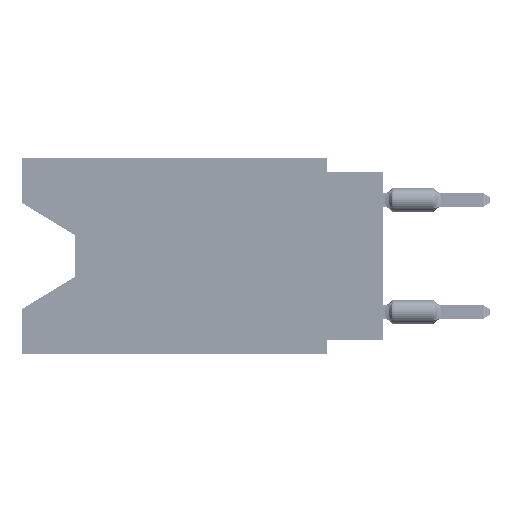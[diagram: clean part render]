
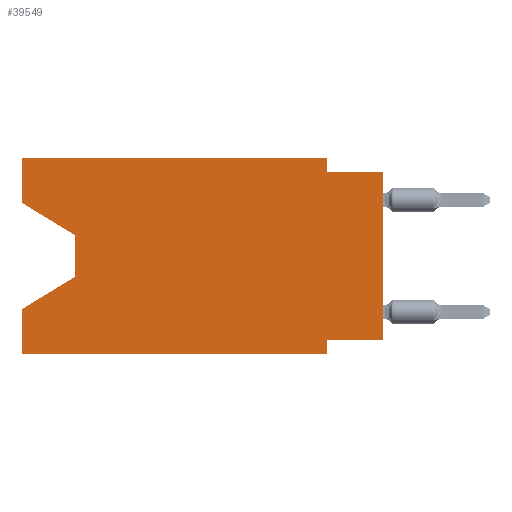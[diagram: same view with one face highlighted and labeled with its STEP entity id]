
A CAD part, left-side view. The second image highlights one B-rep face of the part: STEP entity #39549.
In plain terms, the highlighted planar face has unit normal (-1, 0, 0).
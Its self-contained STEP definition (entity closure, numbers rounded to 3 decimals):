
#186 = CARTESIAN_POINT ( 'NONE',  ( 0., 13.97, -3.505 ) ) ;
#705 = VECTOR ( 'NONE', #32725, 1000. ) ;
#3178 = LINE ( 'NONE', #24293, #705 ) ;
#3574 = EDGE_CURVE ( 'NONE', #90487, #19318, #28671, .T. ) ;
#4982 = LINE ( 'NONE', #40640, #40463 ) ;
#5003 = ORIENTED_EDGE ( 'NONE', *, *, #71803, .F. ) ;
#5248 = VECTOR ( 'NONE', #91007, 1000. ) ;
#5415 = AXIS2_PLACEMENT_3D ( 'NONE', #37842, #21470, #50098 ) ;
#6833 = EDGE_CURVE ( 'NONE', #45487, #69185, #16198, .T. ) ;
#7172 = CARTESIAN_POINT ( 'NONE',  ( 0., 0., 0. ) ) ;
#7627 = DIRECTION ( 'NONE',  ( 0., 0., 1. ) ) ;
#7762 = DIRECTION ( 'NONE',  ( 0., -1., 0. ) ) ;
#8954 = VERTEX_POINT ( 'NONE', #88447 ) ;
#8964 = DIRECTION ( 'NONE',  ( 0., -1., 0. ) ) ;
#9217 = FACE_OUTER_BOUND ( 'NONE', #57411, .T. ) ;
#9561 = CARTESIAN_POINT ( 'NONE',  ( 0., 2.54, 0. ) ) ;
#10021 = CARTESIAN_POINT ( 'NONE',  ( 0., 2.54, -0.635 ) ) ;
#10395 = ORIENTED_EDGE ( 'NONE', *, *, #75110, .F. ) ;
#11474 = CARTESIAN_POINT ( 'NONE',  ( 0., 16.383, -8.89 ) ) ;
#11781 = CARTESIAN_POINT ( 'NONE',  ( 0., 16.383, -2.038 ) ) ;
#15546 = ORIENTED_EDGE ( 'NONE', *, *, #28609, .F. ) ;
#16198 = LINE ( 'NONE', #44834, #74583 ) ;
#16408 = VERTEX_POINT ( 'NONE', #62722 ) ;
#18601 = DIRECTION ( 'NONE',  ( 0., 0., -1. ) ) ;
#19318 = VERTEX_POINT ( 'NONE', #81141 ) ;
#19736 = CARTESIAN_POINT ( 'NONE',  ( 0., 16.383, -2.038 ) ) ;
#19882 = VERTEX_POINT ( 'NONE', #11474 ) ;
#19890 = ORIENTED_EDGE ( 'NONE', *, *, #6833, .F. ) ;
#20108 = VECTOR ( 'NONE', #28737, 1000. ) ;
#21470 = DIRECTION ( 'NONE',  ( 1., 0., 0. ) ) ;
#22603 = ORIENTED_EDGE ( 'NONE', *, *, #80727, .T. ) ;
#24293 = CARTESIAN_POINT ( 'NONE',  ( 0., 2.54, -8.89 ) ) ;
#24719 = CARTESIAN_POINT ( 'NONE',  ( 0., 16.383, 0. ) ) ;
#26148 = DIRECTION ( 'NONE',  ( 0., -1., 0. ) ) ;
#28609 = EDGE_CURVE ( 'NONE', #19882, #33020, #89421, .T. ) ;
#28671 = LINE ( 'NONE', #78869, #62422 ) ;
#28737 = DIRECTION ( 'NONE',  ( 0., 0., 1. ) ) ;
#28832 = ORIENTED_EDGE ( 'NONE', *, *, #74685, .T. ) ;
#29658 = LINE ( 'NONE', #7172, #20108 ) ;
#30761 = DIRECTION ( 'NONE',  ( 0., 1., 0. ) ) ;
#32725 = DIRECTION ( 'NONE',  ( 0., 0., -1. ) ) ;
#33020 = VERTEX_POINT ( 'NONE', #67935 ) ;
#34106 = VECTOR ( 'NONE', #57429, 1000. ) ;
#34855 = VECTOR ( 'NONE', #74922, 1000. ) ;
#37701 = CARTESIAN_POINT ( 'NONE',  ( 0., 16.383, 0. ) ) ;
#37842 = CARTESIAN_POINT ( 'NONE',  ( 0., 16.383, 0. ) ) ;
#39309 = LINE ( 'NONE', #40701, #92547 ) ;
#39549 = ADVANCED_FACE ( 'NONE', ( #9217 ), #43045, .F. ) ;
#40463 = VECTOR ( 'NONE', #18601, 1000. ) ;
#40640 = CARTESIAN_POINT ( 'NONE',  ( 0., 2.54, 0. ) ) ;
#40701 = CARTESIAN_POINT ( 'NONE',  ( 0., 16.383, -8.89 ) ) ;
#41367 = ORIENTED_EDGE ( 'NONE', *, *, #64684, .T. ) ;
#41566 = EDGE_CURVE ( 'NONE', #16408, #19318, #29658, .T. ) ;
#43045 = PLANE ( 'NONE',  #5415 ) ;
#43289 = VERTEX_POINT ( 'NONE', #63779 ) ;
#44834 = CARTESIAN_POINT ( 'NONE',  ( 0., 16.383, 0. ) ) ;
#44967 = LINE ( 'NONE', #89451, #85771 ) ;
#45487 = VERTEX_POINT ( 'NONE', #37701 ) ;
#47924 = VERTEX_POINT ( 'NONE', #75572 ) ;
#50098 = DIRECTION ( 'NONE',  ( 0., 0., -1. ) ) ;
#51078 = ORIENTED_EDGE ( 'NONE', *, *, #81154, .T. ) ;
#51893 = CARTESIAN_POINT ( 'NONE',  ( 0., 0., -8.255 ) ) ;
#55053 = ORIENTED_EDGE ( 'NONE', *, *, #92476, .F. ) ;
#57209 = ORIENTED_EDGE ( 'NONE', *, *, #41566, .T. ) ;
#57383 = LINE ( 'NONE', #63505, #60350 ) ;
#57411 = EDGE_LOOP ( 'NONE', ( #41367, #22603, #28832, #15546, #51078, #55053, #10395, #57209, #88563, #5003, #19890, #90236 ) ) ;
#57429 = DIRECTION ( 'NONE',  ( 0., 0., -1. ) ) ;
#59841 = LINE ( 'NONE', #51893, #63374 ) ;
#60350 = VECTOR ( 'NONE', #7627, 1000. ) ;
#62072 = EDGE_CURVE ( 'NONE', #69712, #45487, #57383, .T. ) ;
#62422 = VECTOR ( 'NONE', #8964, 1000. ) ;
#62722 = CARTESIAN_POINT ( 'NONE',  ( 0., 0., -8.255 ) ) ;
#63371 = LINE ( 'NONE', #11781, #5248 ) ;
#63374 = VECTOR ( 'NONE', #30761, 1000. ) ;
#63505 = CARTESIAN_POINT ( 'NONE',  ( 0., 16.383, 0. ) ) ;
#63779 = CARTESIAN_POINT ( 'NONE',  ( 0., 2.54, -8.255 ) ) ;
#64684 = EDGE_CURVE ( 'NONE', #69712, #47924, #63371, .T. ) ;
#66194 = VERTEX_POINT ( 'NONE', #82506 ) ;
#67910 = DIRECTION ( 'NONE',  ( 0., 0.855, -0.519 ) ) ;
#67935 = CARTESIAN_POINT ( 'NONE',  ( 0., 16.383, -6.852 ) ) ;
#69185 = VERTEX_POINT ( 'NONE', #9561 ) ;
#69712 = VERTEX_POINT ( 'NONE', #19736 ) ;
#71049 = LINE ( 'NONE', #186, #34106 ) ;
#71803 = EDGE_CURVE ( 'NONE', #69185, #90487, #4982, .T. ) ;
#74583 = VECTOR ( 'NONE', #7762, 1000. ) ;
#74685 = EDGE_CURVE ( 'NONE', #66194, #33020, #44967, .T. ) ;
#74922 = DIRECTION ( 'NONE',  ( 0., 0., 1. ) ) ;
#75110 = EDGE_CURVE ( 'NONE', #16408, #43289, #59841, .T. ) ;
#75572 = CARTESIAN_POINT ( 'NONE',  ( 0., 13.97, -3.505 ) ) ;
#78869 = CARTESIAN_POINT ( 'NONE',  ( 0., 0., -0.635 ) ) ;
#80727 = EDGE_CURVE ( 'NONE', #47924, #66194, #71049, .T. ) ;
#81141 = CARTESIAN_POINT ( 'NONE',  ( 0., 0., -0.635 ) ) ;
#81154 = EDGE_CURVE ( 'NONE', #19882, #8954, #39309, .T. ) ;
#82506 = CARTESIAN_POINT ( 'NONE',  ( 0., 13.97, -5.385 ) ) ;
#85771 = VECTOR ( 'NONE', #67910, 1000. ) ;
#88447 = CARTESIAN_POINT ( 'NONE',  ( 0., 2.54, -8.89 ) ) ;
#88563 = ORIENTED_EDGE ( 'NONE', *, *, #3574, .F. ) ;
#89421 = LINE ( 'NONE', #24719, #34855 ) ;
#89451 = CARTESIAN_POINT ( 'NONE',  ( 0., 13.97, -5.385 ) ) ;
#90236 = ORIENTED_EDGE ( 'NONE', *, *, #62072, .F. ) ;
#90487 = VERTEX_POINT ( 'NONE', #10021 ) ;
#91007 = DIRECTION ( 'NONE',  ( 0., -0.855, -0.519 ) ) ;
#92476 = EDGE_CURVE ( 'NONE', #43289, #8954, #3178, .T. ) ;
#92547 = VECTOR ( 'NONE', #26148, 1000. ) ;
